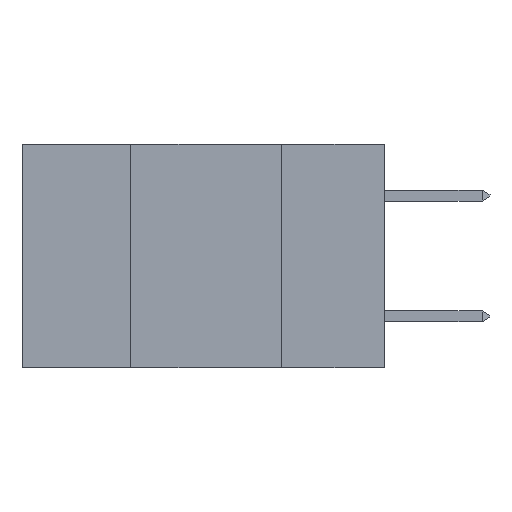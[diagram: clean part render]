
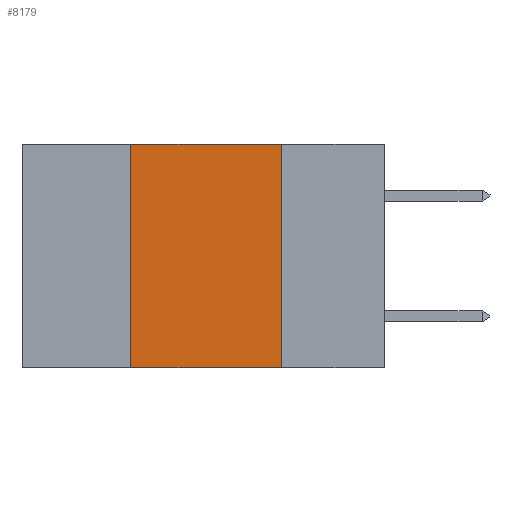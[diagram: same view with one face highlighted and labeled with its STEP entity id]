
A CAD part, left-side view. The second image highlights one B-rep face of the part: STEP entity #8179.
In plain terms, the highlighted planar face has unit normal (-1, 0, 0).
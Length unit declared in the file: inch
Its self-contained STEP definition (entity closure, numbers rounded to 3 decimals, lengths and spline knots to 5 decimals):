
#113 = LINE ( 'NONE', #7684, #7798 ) ;
#240 = VECTOR ( 'NONE', #2384, 39.37008 ) ;
#410 = VERTEX_POINT ( 'NONE', #5370 ) ;
#438 = LINE ( 'NONE', #10314, #3055 ) ;
#474 = ORIENTED_EDGE ( 'NONE', *, *, #3862, .F. ) ;
#875 = LINE ( 'NONE', #6169, #10736 ) ;
#1159 = LINE ( 'NONE', #9051, #240 ) ;
#1654 = EDGE_LOOP ( 'NONE', ( #1701, #9424, #474, #10816 ) ) ;
#1701 = ORIENTED_EDGE ( 'NONE', *, *, #6697, .F. ) ;
#2384 = DIRECTION ( 'NONE',  ( 0., 0., 1. ) ) ;
#3055 = VECTOR ( 'NONE', #6071, 39.37008 ) ;
#3559 = EDGE_CURVE ( 'NONE', #8672, #9135, #113, .T. ) ;
#3862 = EDGE_CURVE ( 'NONE', #5694, #8672, #1159, .T. ) ;
#4212 = CARTESIAN_POINT ( 'NONE',  ( 0., 0.42, 0. ) ) ;
#5370 = CARTESIAN_POINT ( 'NONE',  ( 0., 0.17, -0.37 ) ) ;
#5485 = CARTESIAN_POINT ( 'NONE',  ( 0., 0.17, 0. ) ) ;
#5660 = EDGE_CURVE ( 'NONE', #5694, #410, #875, .T. ) ;
#5694 = VERTEX_POINT ( 'NONE', #7846 ) ;
#6000 = DIRECTION ( 'NONE',  ( 0., -1., 0. ) ) ;
#6028 = DIRECTION ( 'NONE',  ( 0., -1., 0. ) ) ;
#6071 = DIRECTION ( 'NONE',  ( 0., 0., -1. ) ) ;
#6078 = AXIS2_PLACEMENT_3D ( 'NONE', #7682, #7645, #10976 ) ;
#6169 = CARTESIAN_POINT ( 'NONE',  ( 0., 0.6, -0.37 ) ) ;
#6697 = EDGE_CURVE ( 'NONE', #9135, #410, #438, .T. ) ;
#7645 = DIRECTION ( 'NONE',  ( 1., 0., 0. ) ) ;
#7679 = FACE_OUTER_BOUND ( 'NONE', #1654, .T. ) ;
#7682 = CARTESIAN_POINT ( 'NONE',  ( 0., 0.6, 0. ) ) ;
#7684 = CARTESIAN_POINT ( 'NONE',  ( 0., 0.6, 0. ) ) ;
#7722 = PLANE ( 'NONE',  #6078 ) ;
#7798 = VECTOR ( 'NONE', #6028, 39.37008 ) ;
#7846 = CARTESIAN_POINT ( 'NONE',  ( 0., 0.42, -0.37 ) ) ;
#8179 = ADVANCED_FACE ( 'NONE', ( #7679 ), #7722, .F. ) ;
#8672 = VERTEX_POINT ( 'NONE', #4212 ) ;
#9051 = CARTESIAN_POINT ( 'NONE',  ( 0., 0.42, 0. ) ) ;
#9135 = VERTEX_POINT ( 'NONE', #5485 ) ;
#9424 = ORIENTED_EDGE ( 'NONE', *, *, #3559, .F. ) ;
#10314 = CARTESIAN_POINT ( 'NONE',  ( 0., 0.17, 0. ) ) ;
#10736 = VECTOR ( 'NONE', #6000, 39.37008 ) ;
#10816 = ORIENTED_EDGE ( 'NONE', *, *, #5660, .T. ) ;
#10976 = DIRECTION ( 'NONE',  ( 0., 0., -1. ) ) ;
